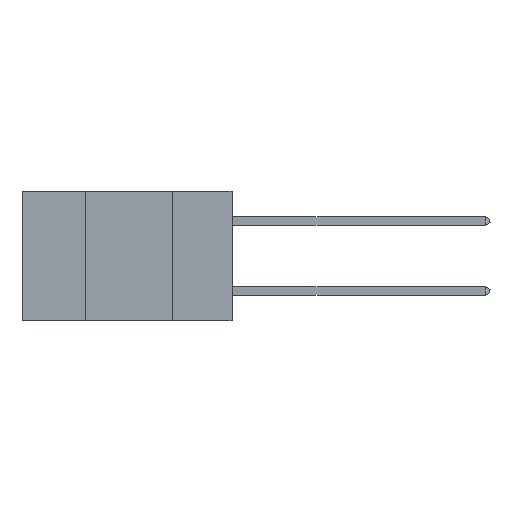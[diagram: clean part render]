
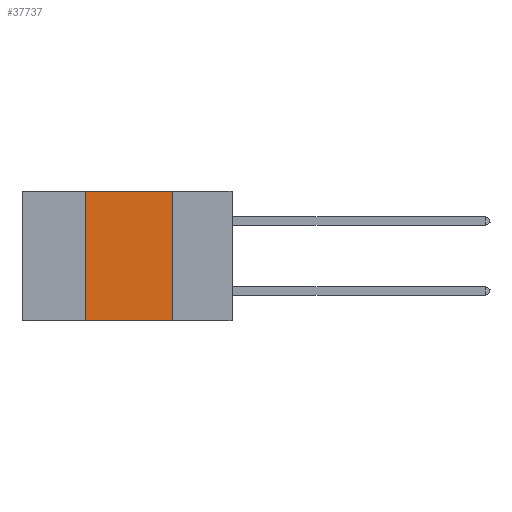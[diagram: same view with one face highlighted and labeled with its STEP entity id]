
A CAD part, left-side view. The second image highlights one B-rep face of the part: STEP entity #37737.
In plain terms, the highlighted planar face has unit normal (-1, 0, 0).
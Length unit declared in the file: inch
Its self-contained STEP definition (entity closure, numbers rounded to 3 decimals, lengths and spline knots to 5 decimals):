
#1385 = EDGE_CURVE ( 'NONE', #19308, #43564, #23424, .T. ) ;
#3108 = ORIENTED_EDGE ( 'NONE', *, *, #26216, .F. ) ;
#3647 = VERTEX_POINT ( 'NONE', #37562 ) ;
#5898 = CARTESIAN_POINT ( 'NONE',  ( 0., 0.17, 0. ) ) ;
#6243 = CARTESIAN_POINT ( 'NONE',  ( 0., 0.6, -0.37 ) ) ;
#7362 = LINE ( 'NONE', #6243, #8486 ) ;
#7727 = EDGE_CURVE ( 'NONE', #3647, #43564, #7362, .T. ) ;
#8318 = DIRECTION ( 'NONE',  ( 0., 0., 1. ) ) ;
#8486 = VECTOR ( 'NONE', #17144, 39.37008 ) ;
#8590 = ORIENTED_EDGE ( 'NONE', *, *, #7727, .T. ) ;
#9253 = EDGE_CURVE ( 'NONE', #9730, #19308, #33808, .T. ) ;
#9574 = DIRECTION ( 'NONE',  ( 1., 0., 0. ) ) ;
#9730 = VERTEX_POINT ( 'NONE', #38518 ) ;
#9743 = PLANE ( 'NONE',  #42039 ) ;
#10297 = CARTESIAN_POINT ( 'NONE',  ( 0., 0.6, 0. ) ) ;
#17144 = DIRECTION ( 'NONE',  ( 0., -1., 0. ) ) ;
#19308 = VERTEX_POINT ( 'NONE', #5898 ) ;
#23166 = CARTESIAN_POINT ( 'NONE',  ( 0., 0.42, 0. ) ) ;
#23424 = LINE ( 'NONE', #37949, #39264 ) ;
#26216 = EDGE_CURVE ( 'NONE', #3647, #9730, #42952, .T. ) ;
#27241 = FACE_OUTER_BOUND ( 'NONE', #35508, .T. ) ;
#27745 = CARTESIAN_POINT ( 'NONE',  ( 0., 0.6, 0. ) ) ;
#28690 = ORIENTED_EDGE ( 'NONE', *, *, #1385, .F. ) ;
#29588 = ORIENTED_EDGE ( 'NONE', *, *, #9253, .F. ) ;
#30391 = VECTOR ( 'NONE', #31601, 39.37008 ) ;
#31601 = DIRECTION ( 'NONE',  ( 0., -1., 0. ) ) ;
#33339 = VECTOR ( 'NONE', #8318, 39.37008 ) ;
#33808 = LINE ( 'NONE', #10297, #30391 ) ;
#33991 = DIRECTION ( 'NONE',  ( 0., 0., -1. ) ) ;
#35508 = EDGE_LOOP ( 'NONE', ( #28690, #29588, #3108, #8590 ) ) ;
#37562 = CARTESIAN_POINT ( 'NONE',  ( 0., 0.42, -0.37 ) ) ;
#37737 = ADVANCED_FACE ( 'NONE', ( #27241 ), #9743, .F. ) ;
#37949 = CARTESIAN_POINT ( 'NONE',  ( 0., 0.17, 0. ) ) ;
#38009 = CARTESIAN_POINT ( 'NONE',  ( 0., 0.17, -0.37 ) ) ;
#38518 = CARTESIAN_POINT ( 'NONE',  ( 0., 0.42, 0. ) ) ;
#39264 = VECTOR ( 'NONE', #33991, 39.37008 ) ;
#42039 = AXIS2_PLACEMENT_3D ( 'NONE', #27745, #9574, #45591 ) ;
#42952 = LINE ( 'NONE', #23166, #33339 ) ;
#43564 = VERTEX_POINT ( 'NONE', #38009 ) ;
#45591 = DIRECTION ( 'NONE',  ( 0., 0., -1. ) ) ;
